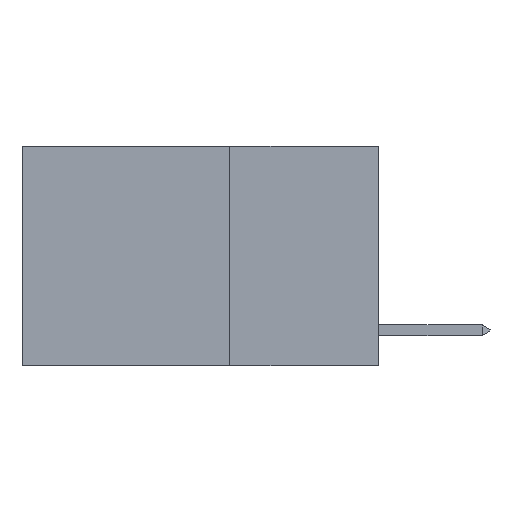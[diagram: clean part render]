
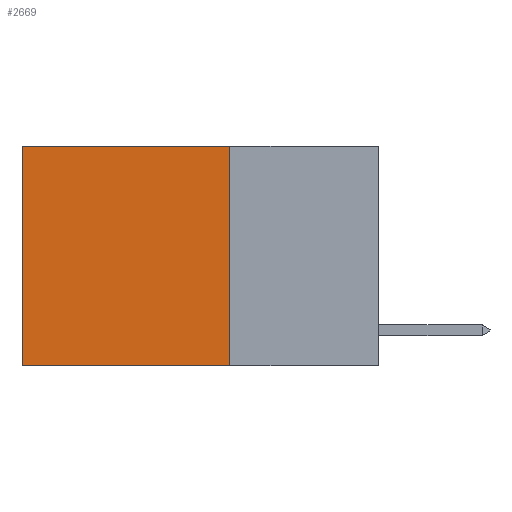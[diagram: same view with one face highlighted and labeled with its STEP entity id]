
A CAD part, left-side view. The second image highlights one B-rep face of the part: STEP entity #2669.
In plain terms, the highlighted planar face has unit normal (-1, 0, 0).
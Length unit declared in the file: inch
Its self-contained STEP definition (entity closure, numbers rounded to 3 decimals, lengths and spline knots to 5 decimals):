
#186 = VERTEX_POINT ( 'NONE', #3005 ) ;
#1439 = FACE_OUTER_BOUND ( 'NONE', #3133, .T. ) ;
#2284 = VECTOR ( 'NONE', #10161, 39.37008 ) ;
#2363 = CARTESIAN_POINT ( 'NONE',  ( 0.2625, 0.25, -0.37 ) ) ;
#2456 = EDGE_CURVE ( 'NONE', #9429, #186, #7948, .T. ) ;
#2669 = ADVANCED_FACE ( 'NONE', ( #1439 ), #8375, .F. ) ;
#3005 = CARTESIAN_POINT ( 'NONE',  ( 0.2625, 0.25, -0.37 ) ) ;
#3133 = EDGE_LOOP ( 'NONE', ( #7593, #7644, #7677, #8131 ) ) ;
#3208 = DIRECTION ( 'NONE',  ( 0., 0., -1. ) ) ;
#3365 = DIRECTION ( 'NONE',  ( 0., 1., 0. ) ) ;
#3863 = VECTOR ( 'NONE', #3365, 39.37008 ) ;
#4013 = CARTESIAN_POINT ( 'NONE',  ( 0.2625, 0.25, 0. ) ) ;
#4245 = VECTOR ( 'NONE', #3208, 39.37008 ) ;
#4261 = VERTEX_POINT ( 'NONE', #8666 ) ;
#4307 = EDGE_CURVE ( 'NONE', #186, #5586, #8579, .T. ) ;
#5586 = VERTEX_POINT ( 'NONE', #7692 ) ;
#5594 = EDGE_CURVE ( 'NONE', #4261, #5586, #6628, .T. ) ;
#6012 = CARTESIAN_POINT ( 'NONE',  ( 0.2625, 0.25, 0. ) ) ;
#6628 = LINE ( 'NONE', #9456, #4245 ) ;
#7026 = EDGE_CURVE ( 'NONE', #9429, #4261, #8964, .T. ) ;
#7593 = ORIENTED_EDGE ( 'NONE', *, *, #5594, .T. ) ;
#7644 = ORIENTED_EDGE ( 'NONE', *, *, #4307, .F. ) ;
#7662 = VECTOR ( 'NONE', #11020, 39.37008 ) ;
#7677 = ORIENTED_EDGE ( 'NONE', *, *, #2456, .F. ) ;
#7692 = CARTESIAN_POINT ( 'NONE',  ( 0.2625, 0.6, -0.37 ) ) ;
#7948 = LINE ( 'NONE', #11104, #7662 ) ;
#8131 = ORIENTED_EDGE ( 'NONE', *, *, #7026, .T. ) ;
#8316 = DIRECTION ( 'NONE',  ( 0., 0., -1. ) ) ;
#8340 = DIRECTION ( 'NONE',  ( 1., 0., 0. ) ) ;
#8365 = CARTESIAN_POINT ( 'NONE',  ( 0.2625, 0.25, 0. ) ) ;
#8375 = PLANE ( 'NONE',  #10675 ) ;
#8579 = LINE ( 'NONE', #2363, #3863 ) ;
#8666 = CARTESIAN_POINT ( 'NONE',  ( 0.2625, 0.6, 0. ) ) ;
#8964 = LINE ( 'NONE', #4013, #2284 ) ;
#9429 = VERTEX_POINT ( 'NONE', #6012 ) ;
#9456 = CARTESIAN_POINT ( 'NONE',  ( 0.2625, 0.6, 0. ) ) ;
#10161 = DIRECTION ( 'NONE',  ( 0., 1., 0. ) ) ;
#10675 = AXIS2_PLACEMENT_3D ( 'NONE', #8365, #8340, #8316 ) ;
#11020 = DIRECTION ( 'NONE',  ( 0., 0., -1. ) ) ;
#11104 = CARTESIAN_POINT ( 'NONE',  ( 0.2625, 0.25, 0. ) ) ;
